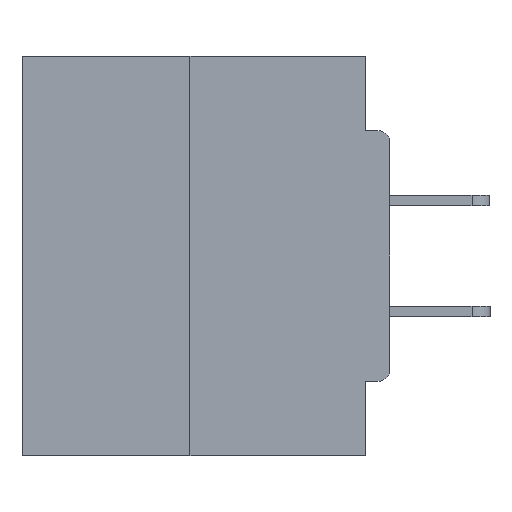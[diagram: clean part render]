
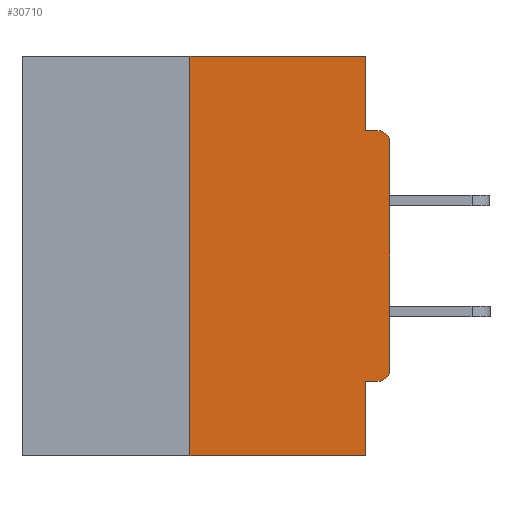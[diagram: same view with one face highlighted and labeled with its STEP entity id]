
A CAD part, left-side view. The second image highlights one B-rep face of the part: STEP entity #30710.
In plain terms, the highlighted planar face has unit normal (-1, 0, 0).
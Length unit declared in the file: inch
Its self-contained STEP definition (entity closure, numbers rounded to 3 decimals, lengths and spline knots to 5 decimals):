
#400 = DIRECTION ( 'NONE',  ( 0., -1., 0. ) ) ;
#877 = ORIENTED_EDGE ( 'NONE', *, *, #3719, .F. ) ;
#1017 = VECTOR ( 'NONE', #34227, 39.37008 ) ;
#1397 = CARTESIAN_POINT ( 'NONE',  ( 0., 0.031, -0.0935 ) ) ;
#1932 = ORIENTED_EDGE ( 'NONE', *, *, #23260, .F. ) ;
#2000 = LINE ( 'NONE', #33544, #19949 ) ;
#2148 = VERTEX_POINT ( 'NONE', #11518 ) ;
#2227 = CARTESIAN_POINT ( 'NONE',  ( 0., 0.015, -0.1085 ) ) ;
#2410 = CARTESIAN_POINT ( 'NONE',  ( 0., 0.031, -0.5 ) ) ;
#2921 = DIRECTION ( 'NONE',  ( 0., 0., -1. ) ) ;
#2952 = CARTESIAN_POINT ( 'NONE',  ( 0., 0.015, -0.3915 ) ) ;
#3049 = EDGE_CURVE ( 'NONE', #8840, #20929, #26656, .T. ) ;
#3719 = EDGE_CURVE ( 'NONE', #5804, #3883, #14803, .T. ) ;
#3764 = CARTESIAN_POINT ( 'NONE',  ( 0., 0.25, 0. ) ) ;
#3883 = VERTEX_POINT ( 'NONE', #3764 ) ;
#4084 = CARTESIAN_POINT ( 'NONE',  ( 0., 0.031, 0. ) ) ;
#4129 = VECTOR ( 'NONE', #400, 39.37008 ) ;
#4982 = VERTEX_POINT ( 'NONE', #1397 ) ;
#5292 = DIRECTION ( 'NONE',  ( 0., 0., -1. ) ) ;
#5804 = VERTEX_POINT ( 'NONE', #35054 ) ;
#8459 = DIRECTION ( 'NONE',  ( -1., 0., 0. ) ) ;
#8840 = VERTEX_POINT ( 'NONE', #22936 ) ;
#8967 = VERTEX_POINT ( 'NONE', #12199 ) ;
#10004 = VERTEX_POINT ( 'NONE', #4084 ) ;
#10439 = LINE ( 'NONE', #2410, #32921 ) ;
#10718 = EDGE_CURVE ( 'NONE', #18360, #26016, #10439, .T. ) ;
#11182 = CARTESIAN_POINT ( 'NONE',  ( 0., 0., -0.3915 ) ) ;
#11281 = LINE ( 'NONE', #17346, #15324 ) ;
#11419 = ORIENTED_EDGE ( 'NONE', *, *, #15807, .T. ) ;
#11518 = CARTESIAN_POINT ( 'NONE',  ( 0., 0.015, -0.0935 ) ) ;
#12199 = CARTESIAN_POINT ( 'NONE',  ( 0., 0., -0.1085 ) ) ;
#12972 = FACE_OUTER_BOUND ( 'NONE', #35817, .T. ) ;
#14001 = DIRECTION ( 'NONE',  ( 1., 0., 0. ) ) ;
#14803 = LINE ( 'NONE', #26543, #31861 ) ;
#14804 = DIRECTION ( 'NONE',  ( 0., 0., 1. ) ) ;
#15324 = VECTOR ( 'NONE', #19967, 39.37008 ) ;
#15581 = ORIENTED_EDGE ( 'NONE', *, *, #17209, .F. ) ;
#15807 = EDGE_CURVE ( 'NONE', #5804, #26016, #11281, .T. ) ;
#16361 = DIRECTION ( 'NONE',  ( 0., 0., -1. ) ) ;
#17027 = PLANE ( 'NONE',  #36446 ) ;
#17209 = EDGE_CURVE ( 'NONE', #8840, #18360, #20311, .T. ) ;
#17340 = AXIS2_PLACEMENT_3D ( 'NONE', #2227, #25162, #16361 ) ;
#17346 = CARTESIAN_POINT ( 'NONE',  ( 0., 0.46, -0.5 ) ) ;
#17535 = EDGE_CURVE ( 'NONE', #8967, #2148, #31011, .T. ) ;
#17716 = CARTESIAN_POINT ( 'NONE',  ( 0., 0.031, -0.5 ) ) ;
#18360 = VERTEX_POINT ( 'NONE', #26638 ) ;
#19949 = VECTOR ( 'NONE', #2921, 39.37008 ) ;
#19967 = DIRECTION ( 'NONE',  ( 0., -1., 0. ) ) ;
#20056 = CARTESIAN_POINT ( 'NONE',  ( 0., 0., -0.0935 ) ) ;
#20311 = LINE ( 'NONE', #31330, #1017 ) ;
#20469 = ORIENTED_EDGE ( 'NONE', *, *, #17535, .T. ) ;
#20929 = VERTEX_POINT ( 'NONE', #11182 ) ;
#21460 = EDGE_CURVE ( 'NONE', #10004, #4982, #2000, .T. ) ;
#22166 = ORIENTED_EDGE ( 'NONE', *, *, #10718, .F. ) ;
#22709 = DIRECTION ( 'NONE',  ( 0., 0., 1. ) ) ;
#22728 = AXIS2_PLACEMENT_3D ( 'NONE', #2952, #8459, #28495 ) ;
#22863 = LINE ( 'NONE', #32042, #30448 ) ;
#22922 = DIRECTION ( 'NONE',  ( 0., 0., -1. ) ) ;
#22936 = CARTESIAN_POINT ( 'NONE',  ( 0., 0.015, -0.4065 ) ) ;
#23260 = EDGE_CURVE ( 'NONE', #4982, #2148, #36863, .T. ) ;
#23353 = CARTESIAN_POINT ( 'NONE',  ( 0., 0., 0. ) ) ;
#25162 = DIRECTION ( 'NONE',  ( -1., 0., 0. ) ) ;
#26016 = VERTEX_POINT ( 'NONE', #17716 ) ;
#26543 = CARTESIAN_POINT ( 'NONE',  ( 0., 0.25, 0. ) ) ;
#26638 = CARTESIAN_POINT ( 'NONE',  ( 0., 0.031, -0.4065 ) ) ;
#26656 = CIRCLE ( 'NONE', #22728, 0.015 ) ;
#28495 = DIRECTION ( 'NONE',  ( 0., 0., -1. ) ) ;
#30448 = VECTOR ( 'NONE', #32662, 39.37008 ) ;
#30685 = VECTOR ( 'NONE', #14804, 39.37008 ) ;
#30710 = ADVANCED_FACE ( 'NONE', ( #12972 ), #17027, .F. ) ;
#30916 = EDGE_CURVE ( 'NONE', #3883, #10004, #22863, .T. ) ;
#31011 = CIRCLE ( 'NONE', #17340, 0.015 ) ;
#31330 = CARTESIAN_POINT ( 'NONE',  ( 0., 0., -0.4065 ) ) ;
#31861 = VECTOR ( 'NONE', #22709, 39.37008 ) ;
#32042 = CARTESIAN_POINT ( 'NONE',  ( 0., 0.46, 0. ) ) ;
#32662 = DIRECTION ( 'NONE',  ( 0., -1., 0. ) ) ;
#32921 = VECTOR ( 'NONE', #5292, 39.37008 ) ;
#32933 = ORIENTED_EDGE ( 'NONE', *, *, #30916, .F. ) ;
#33185 = ORIENTED_EDGE ( 'NONE', *, *, #21460, .F. ) ;
#33544 = CARTESIAN_POINT ( 'NONE',  ( 0., 0.031, 0. ) ) ;
#33989 = ORIENTED_EDGE ( 'NONE', *, *, #34448, .T. ) ;
#34227 = DIRECTION ( 'NONE',  ( 0., 1., 0. ) ) ;
#34448 = EDGE_CURVE ( 'NONE', #20929, #8967, #36528, .T. ) ;
#35054 = CARTESIAN_POINT ( 'NONE',  ( 0., 0.25, -0.5 ) ) ;
#35144 = ORIENTED_EDGE ( 'NONE', *, *, #3049, .T. ) ;
#35817 = EDGE_LOOP ( 'NONE', ( #32933, #877, #11419, #22166, #15581, #35144, #33989, #20469, #1932, #33185 ) ) ;
#36446 = AXIS2_PLACEMENT_3D ( 'NONE', #37093, #14001, #22922 ) ;
#36528 = LINE ( 'NONE', #23353, #30685 ) ;
#36863 = LINE ( 'NONE', #20056, #4129 ) ;
#37093 = CARTESIAN_POINT ( 'NONE',  ( 0., 0.46, 0. ) ) ;
